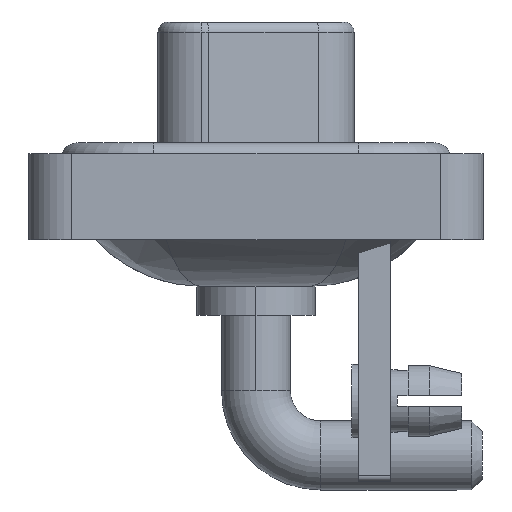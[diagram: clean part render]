
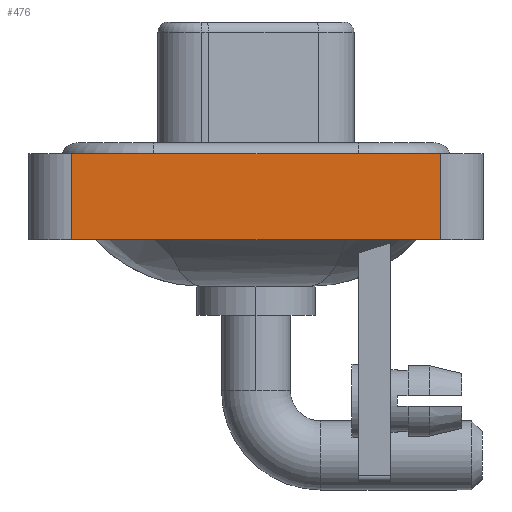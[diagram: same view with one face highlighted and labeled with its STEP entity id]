
A CAD part, left-side view. The second image highlights one B-rep face of the part: STEP entity #476.
In plain terms, the highlighted planar face has unit normal (-1, 0, 0).
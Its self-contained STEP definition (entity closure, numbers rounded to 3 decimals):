
#78 = LINE ( 'NONE', #7783, #6856 ) ;
#476 = ADVANCED_FACE ( 'NONE', ( #17517 ), #18747, .T. ) ;
#719 = DIRECTION ( 'NONE',  ( 0., -1., 0. ) ) ;
#818 = CARTESIAN_POINT ( 'NONE',  ( -7.25, -8.55, -3.6 ) ) ;
#897 = VERTEX_POINT ( 'NONE', #3984 ) ;
#1261 = CARTESIAN_POINT ( 'NONE',  ( -7.25, -8.55, -3.6 ) ) ;
#1612 = CARTESIAN_POINT ( 'NONE',  ( -7.25, -8.55, -3.6 ) ) ;
#3462 = CARTESIAN_POINT ( 'NONE',  ( -7.25, -8.55, 0.4 ) ) ;
#3949 = VERTEX_POINT ( 'NONE', #18776 ) ;
#3984 = CARTESIAN_POINT ( 'NONE',  ( -7.25, 8.55, 0.4 ) ) ;
#4127 = VERTEX_POINT ( 'NONE', #18553 ) ;
#5739 = LINE ( 'NONE', #818, #9717 ) ;
#6571 = DIRECTION ( 'NONE',  ( 0., -1., 0. ) ) ;
#6856 = VECTOR ( 'NONE', #10961, 1000. ) ;
#6966 = ORIENTED_EDGE ( 'NONE', *, *, #15378, .T. ) ;
#7783 = CARTESIAN_POINT ( 'NONE',  ( -7.25, 8.55, -3.6 ) ) ;
#9518 = DIRECTION ( 'NONE',  ( -1., 0., 0. ) ) ;
#9652 = LINE ( 'NONE', #17658, #19666 ) ;
#9717 = VECTOR ( 'NONE', #719, 1000. ) ;
#10961 = DIRECTION ( 'NONE',  ( 0., 0., 1. ) ) ;
#11883 = ORIENTED_EDGE ( 'NONE', *, *, #18266, .T. ) ;
#13252 = VERTEX_POINT ( 'NONE', #3462 ) ;
#13965 = EDGE_LOOP ( 'NONE', ( #6966, #14877, #18715, #11883 ) ) ;
#14119 = DIRECTION ( 'NONE',  ( 0., 0., 1. ) ) ;
#14877 = ORIENTED_EDGE ( 'NONE', *, *, #16303, .F. ) ;
#15143 = EDGE_CURVE ( 'NONE', #4127, #897, #78, .T. ) ;
#15378 = EDGE_CURVE ( 'NONE', #3949, #13252, #18502, .T. ) ;
#15638 = AXIS2_PLACEMENT_3D ( 'NONE', #1612, #9518, #14119 ) ;
#16303 = EDGE_CURVE ( 'NONE', #897, #13252, #9652, .T. ) ;
#16354 = VECTOR ( 'NONE', #18708, 1000. ) ;
#17517 = FACE_OUTER_BOUND ( 'NONE', #13965, .T. ) ;
#17658 = CARTESIAN_POINT ( 'NONE',  ( -7.25, -8.55, 0.4 ) ) ;
#18266 = EDGE_CURVE ( 'NONE', #4127, #3949, #5739, .T. ) ;
#18502 = LINE ( 'NONE', #1261, #16354 ) ;
#18553 = CARTESIAN_POINT ( 'NONE',  ( -7.25, 8.55, -3.6 ) ) ;
#18708 = DIRECTION ( 'NONE',  ( 0., 0., 1. ) ) ;
#18715 = ORIENTED_EDGE ( 'NONE', *, *, #15143, .F. ) ;
#18747 = PLANE ( 'NONE',  #15638 ) ;
#18776 = CARTESIAN_POINT ( 'NONE',  ( -7.25, -8.55, -3.6 ) ) ;
#19666 = VECTOR ( 'NONE', #6571, 1000. ) ;
